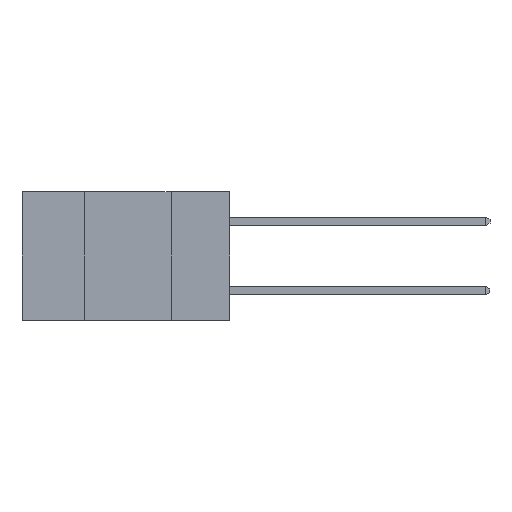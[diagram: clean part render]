
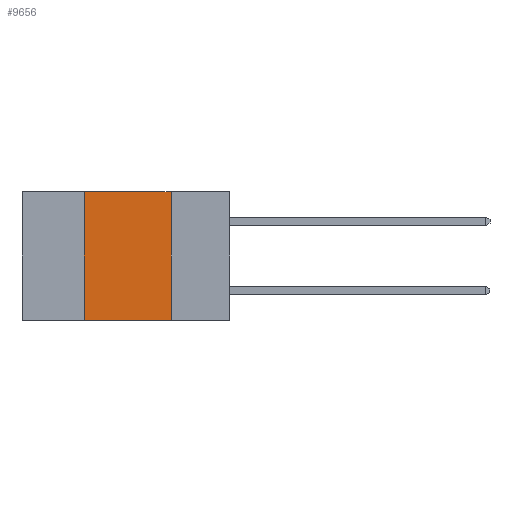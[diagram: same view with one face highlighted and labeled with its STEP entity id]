
A CAD part, left-side view. The second image highlights one B-rep face of the part: STEP entity #9656.
In plain terms, the highlighted planar face has unit normal (-1, 0, 0).
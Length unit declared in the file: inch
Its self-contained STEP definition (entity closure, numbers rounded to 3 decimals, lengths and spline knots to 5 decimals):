
#94 = DIRECTION ( 'NONE',  ( 0., 0., -1. ) ) ;
#111 = CARTESIAN_POINT ( 'NONE',  ( 0., 0.6, -0.37 ) ) ;
#301 = LINE ( 'NONE', #1127, #1290 ) ;
#418 = ORIENTED_EDGE ( 'NONE', *, *, #10630, .F. ) ;
#434 = VERTEX_POINT ( 'NONE', #4222 ) ;
#662 = VECTOR ( 'NONE', #10721, 39.37008 ) ;
#950 = PLANE ( 'NONE',  #3444 ) ;
#1117 = EDGE_CURVE ( 'NONE', #11410, #8003, #6204, .T. ) ;
#1127 = CARTESIAN_POINT ( 'NONE',  ( 0., 0.6, 0. ) ) ;
#1290 = VECTOR ( 'NONE', #2211, 39.37008 ) ;
#1583 = ORIENTED_EDGE ( 'NONE', *, *, #1117, .T. ) ;
#2211 = DIRECTION ( 'NONE',  ( 0., -1., 0. ) ) ;
#2847 = CARTESIAN_POINT ( 'NONE',  ( 0., 0.17, 0. ) ) ;
#3444 = AXIS2_PLACEMENT_3D ( 'NONE', #10200, #11251, #5136 ) ;
#4222 = CARTESIAN_POINT ( 'NONE',  ( 0., 0.17, 0. ) ) ;
#4497 = ORIENTED_EDGE ( 'NONE', *, *, #7618, .F. ) ;
#5136 = DIRECTION ( 'NONE',  ( 0., 0., -1. ) ) ;
#5286 = ORIENTED_EDGE ( 'NONE', *, *, #7774, .F. ) ;
#5840 = DIRECTION ( 'NONE',  ( 0., 0., 1. ) ) ;
#6204 = LINE ( 'NONE', #111, #662 ) ;
#7618 = EDGE_CURVE ( 'NONE', #434, #8003, #12550, .T. ) ;
#7774 = EDGE_CURVE ( 'NONE', #9188, #434, #301, .T. ) ;
#8003 = VERTEX_POINT ( 'NONE', #11289 ) ;
#8188 = CARTESIAN_POINT ( 'NONE',  ( 0., 0.42, -0.37 ) ) ;
#8426 = EDGE_LOOP ( 'NONE', ( #4497, #5286, #418, #1583 ) ) ;
#8949 = CARTESIAN_POINT ( 'NONE',  ( 0., 0.42, 0. ) ) ;
#9103 = LINE ( 'NONE', #8949, #11790 ) ;
#9188 = VERTEX_POINT ( 'NONE', #11223 ) ;
#9656 = ADVANCED_FACE ( 'NONE', ( #10838 ), #950, .F. ) ;
#9853 = VECTOR ( 'NONE', #94, 39.37008 ) ;
#10200 = CARTESIAN_POINT ( 'NONE',  ( 0., 0.6, 0. ) ) ;
#10630 = EDGE_CURVE ( 'NONE', #11410, #9188, #9103, .T. ) ;
#10721 = DIRECTION ( 'NONE',  ( 0., -1., 0. ) ) ;
#10838 = FACE_OUTER_BOUND ( 'NONE', #8426, .T. ) ;
#11223 = CARTESIAN_POINT ( 'NONE',  ( 0., 0.42, 0. ) ) ;
#11251 = DIRECTION ( 'NONE',  ( 1., 0., 0. ) ) ;
#11289 = CARTESIAN_POINT ( 'NONE',  ( 0., 0.17, -0.37 ) ) ;
#11410 = VERTEX_POINT ( 'NONE', #8188 ) ;
#11790 = VECTOR ( 'NONE', #5840, 39.37008 ) ;
#12550 = LINE ( 'NONE', #2847, #9853 ) ;
